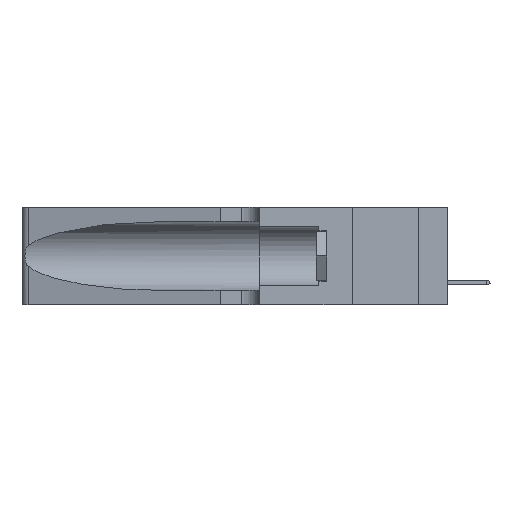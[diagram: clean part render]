
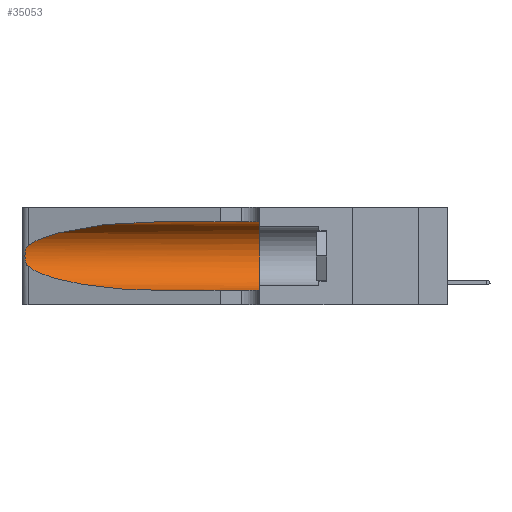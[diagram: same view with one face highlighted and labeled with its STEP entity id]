
A CAD part, left-side view. The second image highlights one B-rep face of the part: STEP entity #35053.
In plain terms, the highlighted cylindrical face has radius 3.308 mm (diameter 6.617 mm), a partial arc.
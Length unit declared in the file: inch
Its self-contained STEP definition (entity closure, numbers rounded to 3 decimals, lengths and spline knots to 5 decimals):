
#412 = VERTEX_POINT ( 'NONE', #9238 ) ;
#495 = CYLINDRICAL_SURFACE ( 'NONE', #28388, 0.13025 ) ;
#498 = CARTESIAN_POINT ( 'NONE',  ( 0.26017, 1.23833, 0.17102 ) ) ;
#651 = CARTESIAN_POINT ( 'NONE',  ( 0.18966, 0.96281, 0.31525 ) ) ;
#2718 = CARTESIAN_POINT ( 'NONE',  ( 0.1305, 1.61858, 0.31525 ) ) ;
#2998 = CARTESIAN_POINT ( 'NONE',  ( 0.1305, 0.72297, 0.05475 ) ) ;
#6445 =( BOUNDED_CURVE ( )  B_SPLINE_CURVE ( 3, ( #23480, #651, #10431, #31128 ),
 .UNSPECIFIED., .F., .F. ) 
 B_SPLINE_CURVE_WITH_KNOTS ( ( 4, 4 ),
 ( 1.5708, 2.84003 ),
 .UNSPECIFIED. ) 
 CURVE ( )  GEOMETRIC_REPRESENTATION_ITEM ( )  RATIONAL_B_SPLINE_CURVE ( ( 1., 0.87, 0.87, 1. ) ) 
 REPRESENTATION_ITEM ( '' )  );
#7194 = EDGE_CURVE ( 'NONE', #412, #21906, #20031, .T. ) ;
#7733 = B_SPLINE_CURVE_WITH_KNOTS ( 'NONE', 3,
 ( #36904, #15577, #21938, #12729, #27509, #24941, #18496, #36630, #498, #21501, #27907, #24665, #24426, #21790 ),
 .UNSPECIFIED., .F., .F.,
 ( 4, 2, 2, 2, 2, 2, 4 ),
 ( 0., 0.00027, 0.00053, 0.00107, 0.0016, 0.00187, 0.00214 ),
 .UNSPECIFIED. ) ;
#7849 = CARTESIAN_POINT ( 'NONE',  ( 0.1305, 0.72297, 0.05475 ) ) ;
#7989 = VERTEX_POINT ( 'NONE', #26653 ) ;
#9238 = CARTESIAN_POINT ( 'NONE',  ( 0.1305, 0.72297, 0.31525 ) ) ;
#9437 = CARTESIAN_POINT ( 'NONE',  ( 0.1305, 0.35, 0.05475 ) ) ;
#9692 = ORIENTED_EDGE ( 'NONE', *, *, #33318, .F. ) ;
#10431 = CARTESIAN_POINT ( 'NONE',  ( 0.2373, 1.15595, 0.28018 ) ) ;
#10914 = FACE_OUTER_BOUND ( 'NONE', #29414, .T. ) ;
#11056 = CIRCLE ( 'NONE', #36562, 0.13025 ) ;
#11109 = ORIENTED_EDGE ( 'NONE', *, *, #26436, .T. ) ;
#12004 = DIRECTION ( 'NONE',  ( 0., -1., 0. ) ) ;
#12729 = CARTESIAN_POINT ( 'NONE',  ( 0.25787, 1.23484, 0.2124 ) ) ;
#13639 = DIRECTION ( 'NONE',  ( 0., -1., 0. ) ) ;
#15577 = CARTESIAN_POINT ( 'NONE',  ( 0.25555, 1.22994, 0.2215 ) ) ;
#15750 = ORIENTED_EDGE ( 'NONE', *, *, #7194, .F. ) ;
#16453 = EDGE_CURVE ( 'NONE', #35328, #30984, #17093, .T. ) ;
#16988 = CARTESIAN_POINT ( 'NONE',  ( 0.18966, 0.96281, 0.05475 ) ) ;
#17093 = LINE ( 'NONE', #34089, #34434 ) ;
#17310 = CARTESIAN_POINT ( 'NONE',  ( 0.1305, 0.35, 0.185 ) ) ;
#18496 = CARTESIAN_POINT ( 'NONE',  ( 0.26075, 1.23896, 0.19203 ) ) ;
#19888 = CARTESIAN_POINT ( 'NONE',  ( 0.2373, 1.15595, 0.08982 ) ) ;
#20031 = LINE ( 'NONE', #2718, #21861 ) ;
#21064 = DIRECTION ( 'NONE',  ( 0., -1., 0. ) ) ;
#21501 = CARTESIAN_POINT ( 'NONE',  ( 0.25856, 1.23593, 0.16098 ) ) ;
#21790 = CARTESIAN_POINT ( 'NONE',  ( 0.25487, 1.22718, 0.14631 ) ) ;
#21861 = VECTOR ( 'NONE', #21064, 39.37008 ) ;
#21906 = VERTEX_POINT ( 'NONE', #33486 ) ;
#21938 = CARTESIAN_POINT ( 'NONE',  ( 0.25639, 1.23184, 0.21858 ) ) ;
#23480 = CARTESIAN_POINT ( 'NONE',  ( 0.1305, 0.72297, 0.31525 ) ) ;
#23832 = ORIENTED_EDGE ( 'NONE', *, *, #31938, .T. ) ;
#24086 = ORIENTED_EDGE ( 'NONE', *, *, #37810, .T. ) ;
#24426 = CARTESIAN_POINT ( 'NONE',  ( 0.25555, 1.22993, 0.14849 ) ) ;
#24665 = CARTESIAN_POINT ( 'NONE',  ( 0.25639, 1.23186, 0.15144 ) ) ;
#24941 = CARTESIAN_POINT ( 'NONE',  ( 0.26018, 1.23835, 0.19895 ) ) ;
#26436 = EDGE_CURVE ( 'NONE', #35337, #35328, #36362, .T. ) ;
#26653 = CARTESIAN_POINT ( 'NONE',  ( 0.25487, 1.22718, 0.22369 ) ) ;
#27509 = CARTESIAN_POINT ( 'NONE',  ( 0.25854, 1.2359, 0.20912 ) ) ;
#27907 = CARTESIAN_POINT ( 'NONE',  ( 0.25789, 1.23486, 0.15765 ) ) ;
#28388 = AXIS2_PLACEMENT_3D ( 'NONE', #30403, #12004, #32985 ) ;
#28810 = DIRECTION ( 'NONE',  ( 0., 1., 0. ) ) ;
#29254 = CARTESIAN_POINT ( 'NONE',  ( 0.25487, 1.22718, 0.14631 ) ) ;
#29414 = EDGE_LOOP ( 'NONE', ( #23832, #24086, #11109, #36397, #9692, #15750 ) ) ;
#30403 = CARTESIAN_POINT ( 'NONE',  ( 0.1305, 1.61858, 0.185 ) ) ;
#30984 = VERTEX_POINT ( 'NONE', #9437 ) ;
#31128 = CARTESIAN_POINT ( 'NONE',  ( 0.25487, 1.22718, 0.22369 ) ) ;
#31923 = CARTESIAN_POINT ( 'NONE',  ( 0.25487, 1.22718, 0.14631 ) ) ;
#31938 = EDGE_CURVE ( 'NONE', #412, #7989, #6445, .T. ) ;
#32985 = DIRECTION ( 'NONE',  ( 0., 0., -1. ) ) ;
#33318 = EDGE_CURVE ( 'NONE', #21906, #30984, #11056, .T. ) ;
#33486 = CARTESIAN_POINT ( 'NONE',  ( 0.1305, 0.35, 0.31525 ) ) ;
#34089 = CARTESIAN_POINT ( 'NONE',  ( 0.1305, 1.61858, 0.05475 ) ) ;
#34434 = VECTOR ( 'NONE', #13639, 39.37008 ) ;
#35053 = ADVANCED_FACE ( 'NONE', ( #10914 ), #495, .F. ) ;
#35328 = VERTEX_POINT ( 'NONE', #7849 ) ;
#35337 = VERTEX_POINT ( 'NONE', #29254 ) ;
#36362 =( BOUNDED_CURVE ( )  B_SPLINE_CURVE ( 3, ( #31923, #19888, #16988, #2998 ),
 .UNSPECIFIED., .F., .F. ) 
 B_SPLINE_CURVE_WITH_KNOTS ( ( 4, 4 ),
 ( 3.44316, 4.71239 ),
 .UNSPECIFIED. ) 
 CURVE ( )  GEOMETRIC_REPRESENTATION_ITEM ( )  RATIONAL_B_SPLINE_CURVE ( ( 1., 0.87, 0.87, 1. ) ) 
 REPRESENTATION_ITEM ( '' )  );
#36397 = ORIENTED_EDGE ( 'NONE', *, *, #16453, .T. ) ;
#36562 = AXIS2_PLACEMENT_3D ( 'NONE', #17310, #28810, #37501 ) ;
#36630 = CARTESIAN_POINT ( 'NONE',  ( 0.26075, 1.23896, 0.178 ) ) ;
#36904 = CARTESIAN_POINT ( 'NONE',  ( 0.25487, 1.22718, 0.22369 ) ) ;
#37501 = DIRECTION ( 'NONE',  ( 0., 0., 1. ) ) ;
#37810 = EDGE_CURVE ( 'NONE', #7989, #35337, #7733, .T. ) ;
